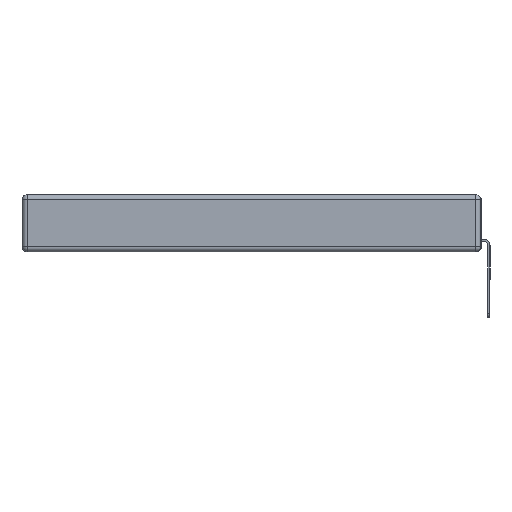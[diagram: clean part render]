
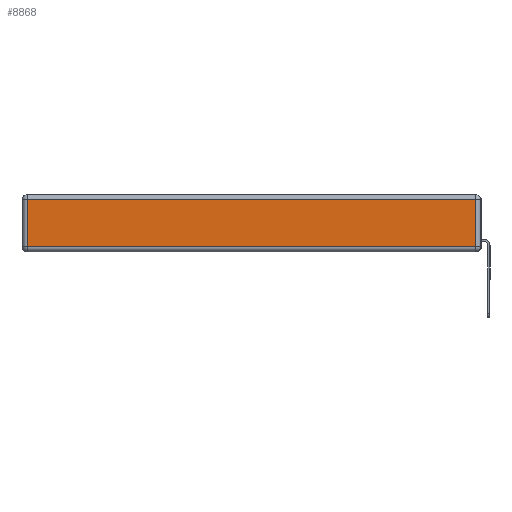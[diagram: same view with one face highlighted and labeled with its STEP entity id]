
A CAD part, left-side view. The second image highlights one B-rep face of the part: STEP entity #8868.
In plain terms, the highlighted planar face has unit normal (-1, 0, 0).
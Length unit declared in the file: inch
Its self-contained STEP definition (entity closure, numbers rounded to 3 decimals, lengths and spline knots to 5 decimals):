
#216 = CARTESIAN_POINT ( 'NONE',  ( 0., 0., -0.313 ) ) ;
#314 = DIRECTION ( 'NONE',  ( 0., 1., 0. ) ) ;
#1379 = CARTESIAN_POINT ( 'NONE',  ( 0., 2.75, -0.03 ) ) ;
#1514 = LINE ( 'NONE', #216, #5693 ) ;
#1865 = ORIENTED_EDGE ( 'NONE', *, *, #15981, .T. ) ;
#2990 = LINE ( 'NONE', #10491, #16047 ) ;
#3169 = PLANE ( 'NONE',  #7275 ) ;
#3395 = EDGE_CURVE ( 'NONE', #15228, #9262, #6508, .T. ) ;
#4307 = CARTESIAN_POINT ( 'NONE',  ( 0., 0., -0.343 ) ) ;
#5693 = VECTOR ( 'NONE', #9015, 39.37008 ) ;
#6369 = EDGE_CURVE ( 'NONE', #11418, #14700, #1514, .T. ) ;
#6508 = LINE ( 'NONE', #1379, #13816 ) ;
#7275 = AXIS2_PLACEMENT_3D ( 'NONE', #4307, #9450, #12878 ) ;
#7782 = LINE ( 'NONE', #9090, #15909 ) ;
#7899 = CARTESIAN_POINT ( 'NONE',  ( 0., 0.03, -0.313 ) ) ;
#8196 = CARTESIAN_POINT ( 'NONE',  ( 0., 0.03, -0.03 ) ) ;
#8868 = ADVANCED_FACE ( 'NONE', ( #11733 ), #3169, .T. ) ;
#9015 = DIRECTION ( 'NONE',  ( 0., -1., 0. ) ) ;
#9090 = CARTESIAN_POINT ( 'NONE',  ( 0., 2.72, -0.343 ) ) ;
#9262 = VERTEX_POINT ( 'NONE', #11538 ) ;
#9450 = DIRECTION ( 'NONE',  ( -1., 0., 0. ) ) ;
#9665 = EDGE_CURVE ( 'NONE', #9262, #11418, #7782, .T. ) ;
#10163 = ORIENTED_EDGE ( 'NONE', *, *, #6369, .T. ) ;
#10491 = CARTESIAN_POINT ( 'NONE',  ( 0., 0.03, -0.343 ) ) ;
#11079 = EDGE_LOOP ( 'NONE', ( #10163, #1865, #11491, #15434 ) ) ;
#11418 = VERTEX_POINT ( 'NONE', #14047 ) ;
#11491 = ORIENTED_EDGE ( 'NONE', *, *, #3395, .T. ) ;
#11538 = CARTESIAN_POINT ( 'NONE',  ( 0., 2.72, -0.03 ) ) ;
#11733 = FACE_OUTER_BOUND ( 'NONE', #11079, .T. ) ;
#11798 = DIRECTION ( 'NONE',  ( 0., 0., 1. ) ) ;
#12878 = DIRECTION ( 'NONE',  ( 0., 0., 1. ) ) ;
#13075 = DIRECTION ( 'NONE',  ( 0., 0., -1. ) ) ;
#13816 = VECTOR ( 'NONE', #314, 39.37008 ) ;
#14047 = CARTESIAN_POINT ( 'NONE',  ( 0., 2.72, -0.313 ) ) ;
#14700 = VERTEX_POINT ( 'NONE', #7899 ) ;
#15228 = VERTEX_POINT ( 'NONE', #8196 ) ;
#15434 = ORIENTED_EDGE ( 'NONE', *, *, #9665, .T. ) ;
#15909 = VECTOR ( 'NONE', #13075, 39.37008 ) ;
#15981 = EDGE_CURVE ( 'NONE', #14700, #15228, #2990, .T. ) ;
#16047 = VECTOR ( 'NONE', #11798, 39.37008 ) ;
